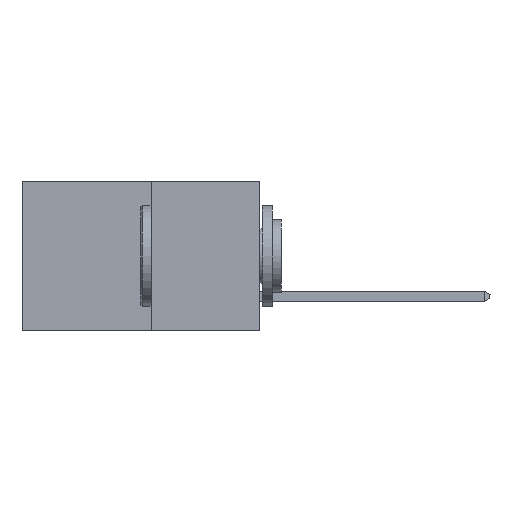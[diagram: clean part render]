
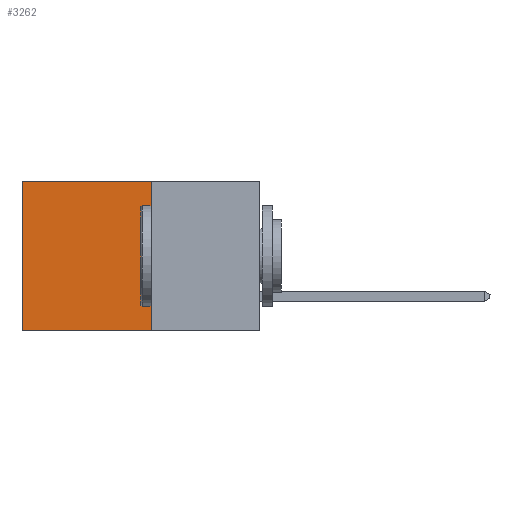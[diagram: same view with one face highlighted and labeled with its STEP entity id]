
A CAD part, left-side view. The second image highlights one B-rep face of the part: STEP entity #3262.
In plain terms, the highlighted planar face has unit normal (-1, 0, 0).
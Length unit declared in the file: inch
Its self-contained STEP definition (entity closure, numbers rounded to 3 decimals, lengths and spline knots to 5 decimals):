
#1266 = EDGE_CURVE ( 'NONE', #3601, #2931, #21863, .T. ) ;
#1607 = VECTOR ( 'NONE', #5771, 39.37008 ) ;
#2211 = CARTESIAN_POINT ( 'NONE',  ( 0.277, 0.27, 0. ) ) ;
#2294 = VECTOR ( 'NONE', #4173, 39.37008 ) ;
#2931 = VERTEX_POINT ( 'NONE', #16970 ) ;
#3262 = ADVANCED_FACE ( 'NONE', ( #22949 ), #4293, .F. ) ;
#3601 = VERTEX_POINT ( 'NONE', #19849 ) ;
#3909 = DIRECTION ( 'NONE',  ( 0., 0., -1. ) ) ;
#4097 = CARTESIAN_POINT ( 'NONE',  ( 0.277, 0.27, -0.37 ) ) ;
#4173 = DIRECTION ( 'NONE',  ( 0., 1., 0. ) ) ;
#4212 = DIRECTION ( 'NONE',  ( 1., 0., 0. ) ) ;
#4293 = PLANE ( 'NONE',  #8722 ) ;
#4551 = VERTEX_POINT ( 'NONE', #8019 ) ;
#5163 = CARTESIAN_POINT ( 'NONE',  ( 0.277, 0.27, -0.37 ) ) ;
#5358 = EDGE_CURVE ( 'NONE', #23381, #4551, #15809, .T. ) ;
#5417 = VECTOR ( 'NONE', #18008, 39.37008 ) ;
#5511 = CARTESIAN_POINT ( 'NONE',  ( 0.277, 0.27, -0.37 ) ) ;
#5771 = DIRECTION ( 'NONE',  ( 0., 0., -1. ) ) ;
#6232 = EDGE_CURVE ( 'NONE', #4551, #2931, #19473, .T. ) ;
#6593 = ORIENTED_EDGE ( 'NONE', *, *, #6232, .F. ) ;
#6921 = EDGE_LOOP ( 'NONE', ( #18091, #6593, #15352, #16165 ) ) ;
#8019 = CARTESIAN_POINT ( 'NONE',  ( 0.277, 0.27, -0.37 ) ) ;
#8722 = AXIS2_PLACEMENT_3D ( 'NONE', #4097, #4212, #3909 ) ;
#12157 = LINE ( 'NONE', #2211, #2294 ) ;
#13358 = VECTOR ( 'NONE', #23798, 39.37008 ) ;
#15352 = ORIENTED_EDGE ( 'NONE', *, *, #5358, .F. ) ;
#15809 = LINE ( 'NONE', #5511, #1607 ) ;
#16165 = ORIENTED_EDGE ( 'NONE', *, *, #17737, .T. ) ;
#16970 = CARTESIAN_POINT ( 'NONE',  ( 0.277, 0.59, -0.37 ) ) ;
#17391 = CARTESIAN_POINT ( 'NONE',  ( 0.277, 0.27, 0. ) ) ;
#17737 = EDGE_CURVE ( 'NONE', #23381, #3601, #12157, .T. ) ;
#18008 = DIRECTION ( 'NONE',  ( 0., 1., 0. ) ) ;
#18091 = ORIENTED_EDGE ( 'NONE', *, *, #1266, .T. ) ;
#19473 = LINE ( 'NONE', #5163, #5417 ) ;
#19849 = CARTESIAN_POINT ( 'NONE',  ( 0.277, 0.59, 0. ) ) ;
#21863 = LINE ( 'NONE', #22322, #13358 ) ;
#22322 = CARTESIAN_POINT ( 'NONE',  ( 0.277, 0.59, -0.37 ) ) ;
#22949 = FACE_OUTER_BOUND ( 'NONE', #6921, .T. ) ;
#23381 = VERTEX_POINT ( 'NONE', #17391 ) ;
#23798 = DIRECTION ( 'NONE',  ( 0., 0., -1. ) ) ;
